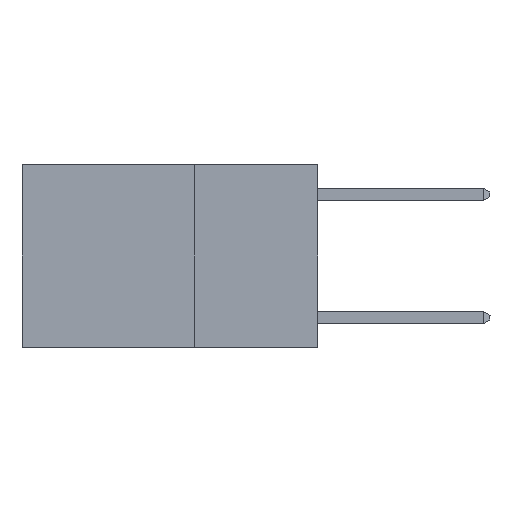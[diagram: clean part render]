
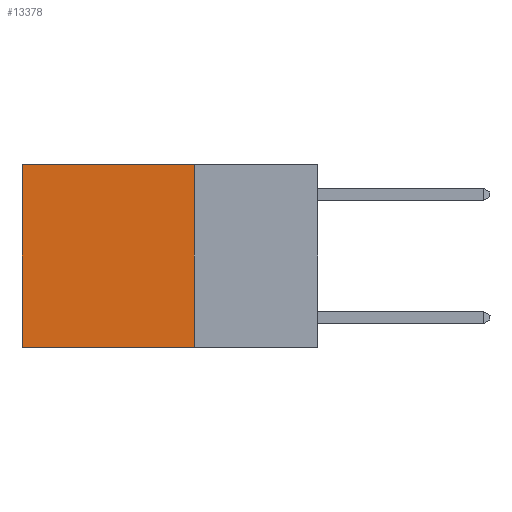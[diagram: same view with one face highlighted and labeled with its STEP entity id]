
A CAD part, left-side view. The second image highlights one B-rep face of the part: STEP entity #13378.
In plain terms, the highlighted planar face has unit normal (-1, 0, 0).
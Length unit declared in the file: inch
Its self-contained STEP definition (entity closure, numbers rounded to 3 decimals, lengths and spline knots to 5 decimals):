
#343 = ORIENTED_EDGE ( 'NONE', *, *, #8860, .F. ) ;
#850 = CARTESIAN_POINT ( 'NONE',  ( 0.2625, 0.25, -0.37 ) ) ;
#1800 = EDGE_CURVE ( 'NONE', #22949, #28387, #25462, .T. ) ;
#2092 = PLANE ( 'NONE',  #26982 ) ;
#2250 = DIRECTION ( 'NONE',  ( 1., 0., 0. ) ) ;
#2847 = CARTESIAN_POINT ( 'NONE',  ( 0.2625, 0.6, 0. ) ) ;
#2921 = ORIENTED_EDGE ( 'NONE', *, *, #21923, .T. ) ;
#3786 = CARTESIAN_POINT ( 'NONE',  ( 0.2625, 0.6, -0.37 ) ) ;
#4481 = CARTESIAN_POINT ( 'NONE',  ( 0.2625, 0.25, 0. ) ) ;
#7047 = VERTEX_POINT ( 'NONE', #4481 ) ;
#8248 = CARTESIAN_POINT ( 'NONE',  ( 0.2625, 0.25, -0.37 ) ) ;
#8694 = EDGE_LOOP ( 'NONE', ( #2921, #11126, #343, #20637 ) ) ;
#8860 = EDGE_CURVE ( 'NONE', #7047, #22949, #29059, .T. ) ;
#11126 = ORIENTED_EDGE ( 'NONE', *, *, #1800, .F. ) ;
#13378 = ADVANCED_FACE ( 'NONE', ( #14085 ), #2092, .F. ) ;
#14085 = FACE_OUTER_BOUND ( 'NONE', #8694, .T. ) ;
#17414 = DIRECTION ( 'NONE',  ( 0., 1., 0. ) ) ;
#18965 = LINE ( 'NONE', #28206, #20627 ) ;
#19110 = CARTESIAN_POINT ( 'NONE',  ( 0.2625, 0.25, 0. ) ) ;
#19532 = VECTOR ( 'NONE', #22577, 39.37008 ) ;
#20627 = VECTOR ( 'NONE', #28519, 39.37008 ) ;
#20637 = ORIENTED_EDGE ( 'NONE', *, *, #23730, .T. ) ;
#21252 = CARTESIAN_POINT ( 'NONE',  ( 0.2625, 0.6, 0. ) ) ;
#21923 = EDGE_CURVE ( 'NONE', #22072, #28387, #25329, .T. ) ;
#22072 = VERTEX_POINT ( 'NONE', #21252 ) ;
#22577 = DIRECTION ( 'NONE',  ( 0., 0., -1. ) ) ;
#22949 = VERTEX_POINT ( 'NONE', #8248 ) ;
#23730 = EDGE_CURVE ( 'NONE', #7047, #22072, #18965, .T. ) ;
#25329 = LINE ( 'NONE', #2847, #19532 ) ;
#25462 = LINE ( 'NONE', #850, #27410 ) ;
#26549 = DIRECTION ( 'NONE',  ( 0., 0., -1. ) ) ;
#26982 = AXIS2_PLACEMENT_3D ( 'NONE', #19110, #2250, #26549 ) ;
#27410 = VECTOR ( 'NONE', #17414, 39.37008 ) ;
#28206 = CARTESIAN_POINT ( 'NONE',  ( 0.2625, 0.25, 0. ) ) ;
#28387 = VERTEX_POINT ( 'NONE', #3786 ) ;
#28519 = DIRECTION ( 'NONE',  ( 0., 1., 0. ) ) ;
#29059 = LINE ( 'NONE', #31328, #31853 ) ;
#29389 = DIRECTION ( 'NONE',  ( 0., 0., -1. ) ) ;
#31328 = CARTESIAN_POINT ( 'NONE',  ( 0.2625, 0.25, 0. ) ) ;
#31853 = VECTOR ( 'NONE', #29389, 39.37008 ) ;
